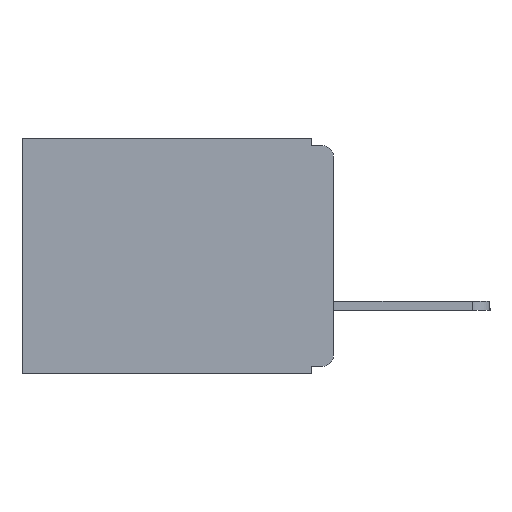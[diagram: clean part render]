
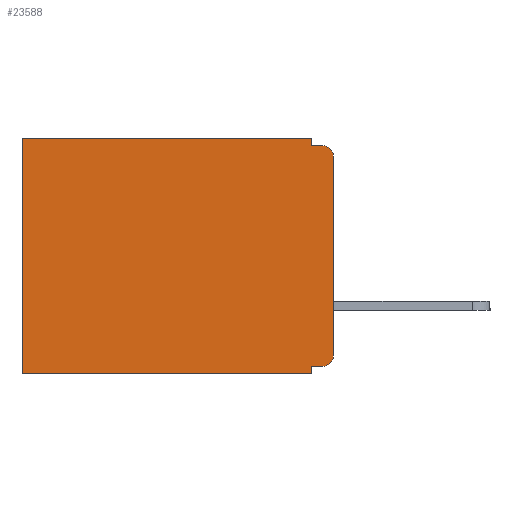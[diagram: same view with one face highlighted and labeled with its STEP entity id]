
A CAD part, left-side view. The second image highlights one B-rep face of the part: STEP entity #23588.
In plain terms, the highlighted planar face has unit normal (-1, 0, 0).
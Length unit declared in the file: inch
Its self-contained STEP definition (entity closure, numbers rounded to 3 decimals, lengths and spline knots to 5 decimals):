
#590 = DIRECTION ( 'NONE',  ( 0., 0., -1. ) ) ;
#1385 = DIRECTION ( 'NONE',  ( 1., 0., 0. ) ) ;
#1501 = CARTESIAN_POINT ( 'NONE',  ( 0.3, 0.015, -0.32 ) ) ;
#2299 = EDGE_CURVE ( 'NONE', #26413, #9553, #20585, .T. ) ;
#2434 = EDGE_LOOP ( 'NONE', ( #15271, #25912, #20811, #12152, #13733, #16072, #10226, #26735, #8272, #14914 ) ) ;
#2925 = CARTESIAN_POINT ( 'NONE',  ( 0.3, 0.031, -0.01 ) ) ;
#3022 = VECTOR ( 'NONE', #13261, 39.37008 ) ;
#3223 = AXIS2_PLACEMENT_3D ( 'NONE', #30638, #15579, #590 ) ;
#3783 = LINE ( 'NONE', #5690, #3022 ) ;
#5205 = VERTEX_POINT ( 'NONE', #2925 ) ;
#5263 = LINE ( 'NONE', #27941, #17842 ) ;
#5690 = CARTESIAN_POINT ( 'NONE',  ( 0.3, 0., -0.01 ) ) ;
#6278 = CARTESIAN_POINT ( 'NONE',  ( 0.3, 0.031, 0. ) ) ;
#6316 = VERTEX_POINT ( 'NONE', #11783 ) ;
#6340 = CARTESIAN_POINT ( 'NONE',  ( 0.3, 0.437, -0.33 ) ) ;
#6405 = CARTESIAN_POINT ( 'NONE',  ( 0.3, 0., -0.33 ) ) ;
#7002 = FACE_OUTER_BOUND ( 'NONE', #2434, .T. ) ;
#7969 = VERTEX_POINT ( 'NONE', #22751 ) ;
#8106 = LINE ( 'NONE', #23564, #28911 ) ;
#8267 = VERTEX_POINT ( 'NONE', #19124 ) ;
#8272 = ORIENTED_EDGE ( 'NONE', *, *, #2299, .F. ) ;
#8555 = DIRECTION ( 'NONE',  ( 0., 1., 0. ) ) ;
#8852 = CARTESIAN_POINT ( 'NONE',  ( 0.3, 0., -0.33 ) ) ;
#9451 = CARTESIAN_POINT ( 'NONE',  ( 0.3, 0.031, -0.33 ) ) ;
#9525 = EDGE_CURVE ( 'NONE', #12688, #5205, #30798, .T. ) ;
#9553 = VERTEX_POINT ( 'NONE', #24314 ) ;
#10226 = ORIENTED_EDGE ( 'NONE', *, *, #14293, .F. ) ;
#11783 = CARTESIAN_POINT ( 'NONE',  ( 0.3, 0., -0.305 ) ) ;
#12152 = ORIENTED_EDGE ( 'NONE', *, *, #9525, .F. ) ;
#12688 = VERTEX_POINT ( 'NONE', #6278 ) ;
#13261 = DIRECTION ( 'NONE',  ( 0., -1., 0. ) ) ;
#13733 = ORIENTED_EDGE ( 'NONE', *, *, #25730, .T. ) ;
#13929 = VECTOR ( 'NONE', #32494, 39.37008 ) ;
#13981 = DIRECTION ( 'NONE',  ( 0., 0., -1. ) ) ;
#14125 = CARTESIAN_POINT ( 'NONE',  ( 0.3, 0.015, -0.025 ) ) ;
#14213 = DIRECTION ( 'NONE',  ( 0., 0., -1. ) ) ;
#14293 = EDGE_CURVE ( 'NONE', #27748, #15134, #5263, .T. ) ;
#14914 = ORIENTED_EDGE ( 'NONE', *, *, #29675, .T. ) ;
#15134 = VERTEX_POINT ( 'NONE', #6340 ) ;
#15271 = ORIENTED_EDGE ( 'NONE', *, *, #26411, .F. ) ;
#15351 = CARTESIAN_POINT ( 'NONE',  ( 0.3, 0.437, 0. ) ) ;
#15542 = CARTESIAN_POINT ( 'NONE',  ( 0.3, 0.031, -0.33 ) ) ;
#15579 = DIRECTION ( 'NONE',  ( -1., 0., 0. ) ) ;
#16072 = ORIENTED_EDGE ( 'NONE', *, *, #32088, .T. ) ;
#16660 = DIRECTION ( 'NONE',  ( 0., 0., -1. ) ) ;
#17012 = DIRECTION ( 'NONE',  ( 0., 0., -1. ) ) ;
#17842 = VECTOR ( 'NONE', #20504, 39.37008 ) ;
#18962 = DIRECTION ( 'NONE',  ( 0., 0., -1. ) ) ;
#19124 = CARTESIAN_POINT ( 'NONE',  ( 0.3, 0.015, -0.01 ) ) ;
#19467 = VECTOR ( 'NONE', #13981, 39.37008 ) ;
#20352 = AXIS2_PLACEMENT_3D ( 'NONE', #8852, #1385, #18962 ) ;
#20504 = DIRECTION ( 'NONE',  ( 0., 1., 0. ) ) ;
#20585 = LINE ( 'NONE', #21279, #26465 ) ;
#20811 = ORIENTED_EDGE ( 'NONE', *, *, #25678, .F. ) ;
#21200 = DIRECTION ( 'NONE',  ( 0., 1., 0. ) ) ;
#21279 = CARTESIAN_POINT ( 'NONE',  ( 0.3, 0., -0.32 ) ) ;
#21354 = PLANE ( 'NONE',  #20352 ) ;
#22751 = CARTESIAN_POINT ( 'NONE',  ( 0.3, 0., -0.025 ) ) ;
#23564 = CARTESIAN_POINT ( 'NONE',  ( 0.3, 0., 0. ) ) ;
#23588 = ADVANCED_FACE ( 'NONE', ( #7002 ), #21354, .F. ) ;
#23736 = VERTEX_POINT ( 'NONE', #15351 ) ;
#24314 = CARTESIAN_POINT ( 'NONE',  ( 0.3, 0.031, -0.32 ) ) ;
#25340 = EDGE_CURVE ( 'NONE', #9553, #27748, #31683, .T. ) ;
#25678 = EDGE_CURVE ( 'NONE', #5205, #8267, #3783, .T. ) ;
#25730 = EDGE_CURVE ( 'NONE', #12688, #23736, #8106, .T. ) ;
#25912 = ORIENTED_EDGE ( 'NONE', *, *, #29943, .T. ) ;
#26411 = EDGE_CURVE ( 'NONE', #7969, #6316, #27706, .T. ) ;
#26413 = VERTEX_POINT ( 'NONE', #1501 ) ;
#26465 = VECTOR ( 'NONE', #21200, 39.37008 ) ;
#26735 = ORIENTED_EDGE ( 'NONE', *, *, #25340, .F. ) ;
#26774 = CARTESIAN_POINT ( 'NONE',  ( 0.3, 0.031, 0. ) ) ;
#27317 = LINE ( 'NONE', #27493, #13929 ) ;
#27467 = CIRCLE ( 'NONE', #30133, 0.015 ) ;
#27493 = CARTESIAN_POINT ( 'NONE',  ( 0.3, 0.437, -0.33 ) ) ;
#27706 = LINE ( 'NONE', #6405, #19467 ) ;
#27748 = VERTEX_POINT ( 'NONE', #15542 ) ;
#27871 = CIRCLE ( 'NONE', #3223, 0.015 ) ;
#27941 = CARTESIAN_POINT ( 'NONE',  ( 0.3, 0., -0.33 ) ) ;
#28911 = VECTOR ( 'NONE', #8555, 39.37008 ) ;
#29675 = EDGE_CURVE ( 'NONE', #26413, #6316, #27871, .T. ) ;
#29943 = EDGE_CURVE ( 'NONE', #7969, #8267, #27467, .T. ) ;
#30133 = AXIS2_PLACEMENT_3D ( 'NONE', #14125, #31699, #16660 ) ;
#30638 = CARTESIAN_POINT ( 'NONE',  ( 0.3, 0.015, -0.305 ) ) ;
#30798 = LINE ( 'NONE', #26774, #31585 ) ;
#30888 = VECTOR ( 'NONE', #17012, 39.37008 ) ;
#31585 = VECTOR ( 'NONE', #14213, 39.37008 ) ;
#31683 = LINE ( 'NONE', #9451, #30888 ) ;
#31699 = DIRECTION ( 'NONE',  ( -1., 0., 0. ) ) ;
#32088 = EDGE_CURVE ( 'NONE', #23736, #15134, #27317, .T. ) ;
#32494 = DIRECTION ( 'NONE',  ( 0., 0., -1. ) ) ;
